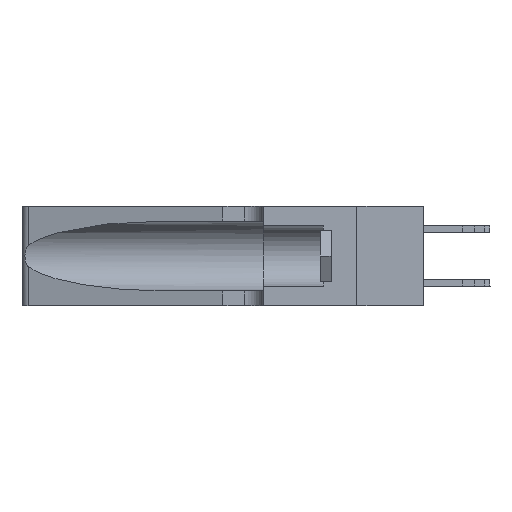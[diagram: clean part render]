
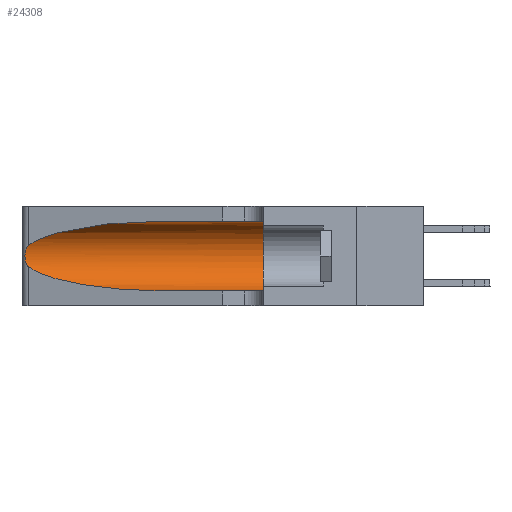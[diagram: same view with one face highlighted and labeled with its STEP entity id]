
A CAD part, left-side view. The second image highlights one B-rep face of the part: STEP entity #24308.
In plain terms, the highlighted cylindrical face has radius 3.308 mm (diameter 6.617 mm), a partial arc.
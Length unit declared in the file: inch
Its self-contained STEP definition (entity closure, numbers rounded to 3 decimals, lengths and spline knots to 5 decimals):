
#21 = CARTESIAN_POINT ( 'NONE',  ( 0.25487, 1.22718, 0.14631 ) ) ;
#256 = CARTESIAN_POINT ( 'NONE',  ( 0.26018, 1.23835, 0.19895 ) ) ;
#410 = ORIENTED_EDGE ( 'NONE', *, *, #23749, .T. ) ;
#2239 = EDGE_CURVE ( 'NONE', #11173, #14397, #13447, .T. ) ;
#2253 = CARTESIAN_POINT ( 'NONE',  ( 0.25787, 1.23484, 0.2124 ) ) ;
#2478 = CARTESIAN_POINT ( 'NONE',  ( 0.1305, 0.35, 0.05475 ) ) ;
#2836 = DIRECTION ( 'NONE',  ( 0., -1., 0. ) ) ;
#3084 = EDGE_LOOP ( 'NONE', ( #27639, #21143, #410, #12001, #5686, #22563 ) ) ;
#4133 = VERTEX_POINT ( 'NONE', #5042 ) ;
#4265 = EDGE_CURVE ( 'NONE', #4133, #27774, #21884, .T. ) ;
#5042 = CARTESIAN_POINT ( 'NONE',  ( 0.1305, 0.72297, 0.31525 ) ) ;
#5686 = ORIENTED_EDGE ( 'NONE', *, *, #20985, .F. ) ;
#6938 = LINE ( 'NONE', #18123, #12643 ) ;
#7765 = VECTOR ( 'NONE', #11697, 39.37008 ) ;
#9783 = CYLINDRICAL_SURFACE ( 'NONE', #19121, 0.13025 ) ;
#10632 = DIRECTION ( 'NONE',  ( 0., 1., 0. ) ) ;
#10714 = CARTESIAN_POINT ( 'NONE',  ( 0.25487, 1.22718, 0.22369 ) ) ;
#10894 = CARTESIAN_POINT ( 'NONE',  ( 0.25639, 1.23184, 0.21858 ) ) ;
#10942 =( BOUNDED_CURVE ( )  B_SPLINE_CURVE ( 3, ( #19480, #21499, #13044, #23660 ),
 .UNSPECIFIED., .F., .F. ) 
 B_SPLINE_CURVE_WITH_KNOTS ( ( 4, 4 ),
 ( 3.44316, 4.71239 ),
 .UNSPECIFIED. ) 
 CURVE ( )  GEOMETRIC_REPRESENTATION_ITEM ( )  RATIONAL_B_SPLINE_CURVE ( ( 1., 0.87, 0.87, 1. ) ) 
 REPRESENTATION_ITEM ( '' )  );
#11173 = VERTEX_POINT ( 'NONE', #11496 ) ;
#11294 = DIRECTION ( 'NONE',  ( 0., 0., -1. ) ) ;
#11496 = CARTESIAN_POINT ( 'NONE',  ( 0.1305, 0.72297, 0.05475 ) ) ;
#11697 = DIRECTION ( 'NONE',  ( 0., -1., 0. ) ) ;
#12001 = ORIENTED_EDGE ( 'NONE', *, *, #2239, .T. ) ;
#12643 = VECTOR ( 'NONE', #26426, 39.37008 ) ;
#13044 = CARTESIAN_POINT ( 'NONE',  ( 0.18966, 0.96281, 0.05475 ) ) ;
#13058 = CARTESIAN_POINT ( 'NONE',  ( 0.25856, 1.23593, 0.16098 ) ) ;
#13447 = LINE ( 'NONE', #24464, #7765 ) ;
#13723 = VERTEX_POINT ( 'NONE', #14012 ) ;
#14012 = CARTESIAN_POINT ( 'NONE',  ( 0.25487, 1.22718, 0.14631 ) ) ;
#14397 = VERTEX_POINT ( 'NONE', #2478 ) ;
#15404 = CARTESIAN_POINT ( 'NONE',  ( 0.25555, 1.22993, 0.14849 ) ) ;
#15534 = CARTESIAN_POINT ( 'NONE',  ( 0.2373, 1.15595, 0.28018 ) ) ;
#16155 = AXIS2_PLACEMENT_3D ( 'NONE', #25655, #10632, #27828 ) ;
#17313 = CARTESIAN_POINT ( 'NONE',  ( 0.25789, 1.23486, 0.15765 ) ) ;
#17912 = CARTESIAN_POINT ( 'NONE',  ( 0.18966, 0.96281, 0.31525 ) ) ;
#17933 = EDGE_CURVE ( 'NONE', #4133, #26089, #6938, .T. ) ;
#18057 = B_SPLINE_CURVE_WITH_KNOTS ( 'NONE', 3,
 ( #10714, #23394, #10894, #2253, #26197, #256, #19494, #21882, #23854, #13058, #17313, #26001, #15404, #21 ),
 .UNSPECIFIED., .F., .F.,
 ( 4, 2, 2, 2, 2, 2, 4 ),
 ( 0., 0.00027, 0.00053, 0.00107, 0.0016, 0.00187, 0.00214 ),
 .UNSPECIFIED. ) ;
#18103 = CARTESIAN_POINT ( 'NONE',  ( 0.1305, 1.61858, 0.185 ) ) ;
#18123 = CARTESIAN_POINT ( 'NONE',  ( 0.1305, 1.61858, 0.31525 ) ) ;
#19121 = AXIS2_PLACEMENT_3D ( 'NONE', #18103, #2836, #11294 ) ;
#19414 = CIRCLE ( 'NONE', #16155, 0.13025 ) ;
#19480 = CARTESIAN_POINT ( 'NONE',  ( 0.25487, 1.22718, 0.14631 ) ) ;
#19494 = CARTESIAN_POINT ( 'NONE',  ( 0.26075, 1.23896, 0.19203 ) ) ;
#20985 = EDGE_CURVE ( 'NONE', #26089, #14397, #19414, .T. ) ;
#21143 = ORIENTED_EDGE ( 'NONE', *, *, #26622, .T. ) ;
#21499 = CARTESIAN_POINT ( 'NONE',  ( 0.2373, 1.15595, 0.08982 ) ) ;
#21882 = CARTESIAN_POINT ( 'NONE',  ( 0.26075, 1.23896, 0.178 ) ) ;
#21884 =( BOUNDED_CURVE ( )  B_SPLINE_CURVE ( 3, ( #22089, #17912, #15534, #26405 ),
 .UNSPECIFIED., .F., .T. ) 
 B_SPLINE_CURVE_WITH_KNOTS ( ( 4, 4 ),
 ( 1.5708, 2.84003 ),
 .UNSPECIFIED. ) 
 CURVE ( )  GEOMETRIC_REPRESENTATION_ITEM ( )  RATIONAL_B_SPLINE_CURVE ( ( 1., 0.87, 0.87, 1. ) ) 
 REPRESENTATION_ITEM ( '' )  );
#21943 = FACE_OUTER_BOUND ( 'NONE', #3084, .T. ) ;
#22089 = CARTESIAN_POINT ( 'NONE',  ( 0.1305, 0.72297, 0.31525 ) ) ;
#22563 = ORIENTED_EDGE ( 'NONE', *, *, #17933, .F. ) ;
#23394 = CARTESIAN_POINT ( 'NONE',  ( 0.25555, 1.22994, 0.2215 ) ) ;
#23660 = CARTESIAN_POINT ( 'NONE',  ( 0.1305, 0.72297, 0.05475 ) ) ;
#23749 = EDGE_CURVE ( 'NONE', #13723, #11173, #10942, .T. ) ;
#23854 = CARTESIAN_POINT ( 'NONE',  ( 0.26017, 1.23833, 0.17102 ) ) ;
#24060 = CARTESIAN_POINT ( 'NONE',  ( 0.1305, 0.35, 0.31525 ) ) ;
#24308 = ADVANCED_FACE ( 'NONE', ( #21943 ), #9783, .F. ) ;
#24464 = CARTESIAN_POINT ( 'NONE',  ( 0.1305, 1.61858, 0.05475 ) ) ;
#25655 = CARTESIAN_POINT ( 'NONE',  ( 0.1305, 0.35, 0.185 ) ) ;
#25723 = CARTESIAN_POINT ( 'NONE',  ( 0.25487, 1.22718, 0.22369 ) ) ;
#26001 = CARTESIAN_POINT ( 'NONE',  ( 0.25639, 1.23186, 0.15144 ) ) ;
#26089 = VERTEX_POINT ( 'NONE', #24060 ) ;
#26197 = CARTESIAN_POINT ( 'NONE',  ( 0.25854, 1.2359, 0.20912 ) ) ;
#26405 = CARTESIAN_POINT ( 'NONE',  ( 0.25487, 1.22718, 0.22369 ) ) ;
#26426 = DIRECTION ( 'NONE',  ( 0., -1., 0. ) ) ;
#26622 = EDGE_CURVE ( 'NONE', #27774, #13723, #18057, .T. ) ;
#27639 = ORIENTED_EDGE ( 'NONE', *, *, #4265, .T. ) ;
#27774 = VERTEX_POINT ( 'NONE', #25723 ) ;
#27828 = DIRECTION ( 'NONE',  ( 0., 0., 1. ) ) ;
